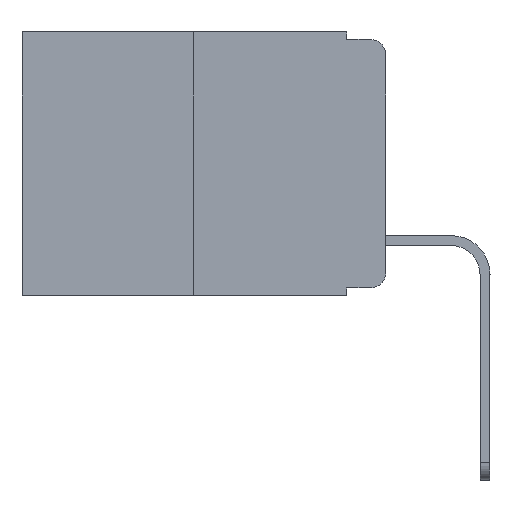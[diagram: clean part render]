
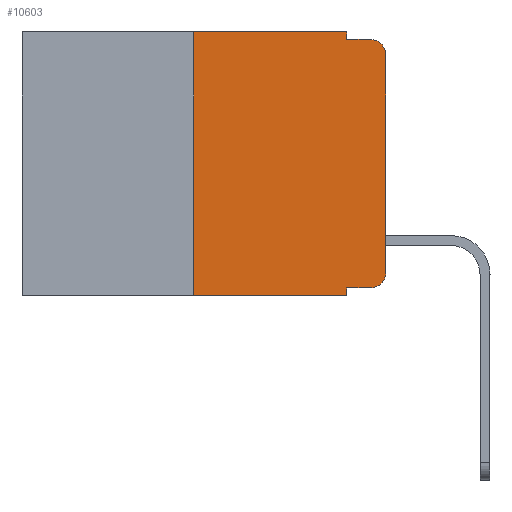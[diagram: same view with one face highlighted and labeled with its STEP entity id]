
A CAD part, left-side view. The second image highlights one B-rep face of the part: STEP entity #10603.
In plain terms, the highlighted planar face has unit normal (-1, 0, 0).
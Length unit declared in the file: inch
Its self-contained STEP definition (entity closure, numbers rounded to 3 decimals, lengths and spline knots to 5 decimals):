
#45 = DIRECTION ( 'NONE',  ( 1., 0., 0. ) ) ;
#70 = CARTESIAN_POINT ( 'NONE',  ( 0., 0.051, -0.343 ) ) ;
#143 = DIRECTION ( 'NONE',  ( 0., 0., -1. ) ) ;
#211 = VECTOR ( 'NONE', #8618, 39.37008 ) ;
#401 = EDGE_CURVE ( 'NONE', #9025, #5847, #8003, .T. ) ;
#471 = CARTESIAN_POINT ( 'NONE',  ( 0., 0.25, 0. ) ) ;
#482 = LINE ( 'NONE', #4358, #211 ) ;
#632 = ORIENTED_EDGE ( 'NONE', *, *, #1402, .T. ) ;
#635 = VERTEX_POINT ( 'NONE', #2144 ) ;
#661 = VECTOR ( 'NONE', #1377, 39.37008 ) ;
#1080 = EDGE_CURVE ( 'NONE', #9693, #635, #1495, .T. ) ;
#1377 = DIRECTION ( 'NONE',  ( 0., 0., 1. ) ) ;
#1402 = EDGE_CURVE ( 'NONE', #5847, #8115, #1760, .T. ) ;
#1495 = LINE ( 'NONE', #10605, #9600 ) ;
#1736 = ORIENTED_EDGE ( 'NONE', *, *, #7422, .F. ) ;
#1760 = LINE ( 'NONE', #5033, #10663 ) ;
#1771 = CARTESIAN_POINT ( 'NONE',  ( 0., 0.473, 0. ) ) ;
#1972 = DIRECTION ( 'NONE',  ( -1., 0., 0. ) ) ;
#2054 = LINE ( 'NONE', #2616, #4363 ) ;
#2144 = CARTESIAN_POINT ( 'NONE',  ( 0., 0.02, -0.01 ) ) ;
#2616 = CARTESIAN_POINT ( 'NONE',  ( 0., 0.051, -0.333 ) ) ;
#2675 = EDGE_LOOP ( 'NONE', ( #632, #10513, #5081, #4228, #2771, #8760, #10245, #1736, #8537, #11148 ) ) ;
#2734 = EDGE_CURVE ( 'NONE', #5361, #9025, #2054, .T. ) ;
#2771 = ORIENTED_EDGE ( 'NONE', *, *, #8094, .F. ) ;
#2781 = EDGE_CURVE ( 'NONE', #10192, #9693, #7338, .T. ) ;
#2884 = AXIS2_PLACEMENT_3D ( 'NONE', #5532, #1972, #4721 ) ;
#2901 = LINE ( 'NONE', #6798, #3985 ) ;
#3283 = FACE_OUTER_BOUND ( 'NONE', #2675, .T. ) ;
#3798 = CARTESIAN_POINT ( 'NONE',  ( 0., 0.02, -0.333 ) ) ;
#3841 = CARTESIAN_POINT ( 'NONE',  ( 0., 0.051, 0. ) ) ;
#3880 = VERTEX_POINT ( 'NONE', #7489 ) ;
#3985 = VECTOR ( 'NONE', #10196, 39.37008 ) ;
#4228 = ORIENTED_EDGE ( 'NONE', *, *, #2781, .F. ) ;
#4239 = CIRCLE ( 'NONE', #2884, 0.02 ) ;
#4358 = CARTESIAN_POINT ( 'NONE',  ( 0., 0.051, 0. ) ) ;
#4363 = VECTOR ( 'NONE', #6846, 39.37008 ) ;
#4426 = DIRECTION ( 'NONE',  ( 0., -1., 0. ) ) ;
#4572 = DIRECTION ( 'NONE',  ( -1., 0., 0. ) ) ;
#4721 = DIRECTION ( 'NONE',  ( 0., 0., -1. ) ) ;
#5033 = CARTESIAN_POINT ( 'NONE',  ( 0., 0., 0. ) ) ;
#5081 = ORIENTED_EDGE ( 'NONE', *, *, #1080, .F. ) ;
#5195 = CARTESIAN_POINT ( 'NONE',  ( 0., 0.051, -0.333 ) ) ;
#5239 = AXIS2_PLACEMENT_3D ( 'NONE', #10438, #4572, #143 ) ;
#5260 = VERTEX_POINT ( 'NONE', #70 ) ;
#5361 = VERTEX_POINT ( 'NONE', #5195 ) ;
#5532 = CARTESIAN_POINT ( 'NONE',  ( 0., 0.02, -0.03 ) ) ;
#5631 = EDGE_CURVE ( 'NONE', #9500, #3880, #8090, .T. ) ;
#5632 = VECTOR ( 'NONE', #4426, 39.37008 ) ;
#5847 = VERTEX_POINT ( 'NONE', #8410 ) ;
#6134 = CARTESIAN_POINT ( 'NONE',  ( 0., 0.473, 0. ) ) ;
#6629 = CARTESIAN_POINT ( 'NONE',  ( 0., 0.051, -0.01 ) ) ;
#6798 = CARTESIAN_POINT ( 'NONE',  ( 0., 0.473, -0.343 ) ) ;
#6846 = DIRECTION ( 'NONE',  ( 0., -1., 0. ) ) ;
#6994 = CARTESIAN_POINT ( 'NONE',  ( 0., 0.051, 0. ) ) ;
#7025 = DIRECTION ( 'NONE',  ( 0., 0., -1. ) ) ;
#7338 = LINE ( 'NONE', #6994, #9633 ) ;
#7422 = EDGE_CURVE ( 'NONE', #5361, #5260, #482, .T. ) ;
#7489 = CARTESIAN_POINT ( 'NONE',  ( 0., 0.25, 0. ) ) ;
#8003 = CIRCLE ( 'NONE', #5239, 0.02 ) ;
#8090 = LINE ( 'NONE', #471, #661 ) ;
#8094 = EDGE_CURVE ( 'NONE', #3880, #10192, #9415, .T. ) ;
#8115 = VERTEX_POINT ( 'NONE', #8641 ) ;
#8198 = AXIS2_PLACEMENT_3D ( 'NONE', #1771, #45, #8721 ) ;
#8410 = CARTESIAN_POINT ( 'NONE',  ( 0., 0., -0.313 ) ) ;
#8537 = ORIENTED_EDGE ( 'NONE', *, *, #2734, .T. ) ;
#8578 = EDGE_CURVE ( 'NONE', #9500, #5260, #2901, .T. ) ;
#8618 = DIRECTION ( 'NONE',  ( 0., 0., -1. ) ) ;
#8641 = CARTESIAN_POINT ( 'NONE',  ( 0., 0., -0.03 ) ) ;
#8721 = DIRECTION ( 'NONE',  ( 0., 0., -1. ) ) ;
#8760 = ORIENTED_EDGE ( 'NONE', *, *, #5631, .F. ) ;
#9025 = VERTEX_POINT ( 'NONE', #3798 ) ;
#9415 = LINE ( 'NONE', #6134, #5632 ) ;
#9500 = VERTEX_POINT ( 'NONE', #10623 ) ;
#9525 = EDGE_CURVE ( 'NONE', #8115, #635, #4239, .T. ) ;
#9600 = VECTOR ( 'NONE', #10647, 39.37008 ) ;
#9633 = VECTOR ( 'NONE', #7025, 39.37008 ) ;
#9693 = VERTEX_POINT ( 'NONE', #6629 ) ;
#10192 = VERTEX_POINT ( 'NONE', #3841 ) ;
#10196 = DIRECTION ( 'NONE',  ( 0., -1., 0. ) ) ;
#10213 = DIRECTION ( 'NONE',  ( 0., 0., 1. ) ) ;
#10245 = ORIENTED_EDGE ( 'NONE', *, *, #8578, .T. ) ;
#10416 = PLANE ( 'NONE',  #8198 ) ;
#10438 = CARTESIAN_POINT ( 'NONE',  ( 0., 0.02, -0.313 ) ) ;
#10513 = ORIENTED_EDGE ( 'NONE', *, *, #9525, .T. ) ;
#10603 = ADVANCED_FACE ( 'NONE', ( #3283 ), #10416, .F. ) ;
#10605 = CARTESIAN_POINT ( 'NONE',  ( 0., 0.051, -0.01 ) ) ;
#10623 = CARTESIAN_POINT ( 'NONE',  ( 0., 0.25, -0.343 ) ) ;
#10647 = DIRECTION ( 'NONE',  ( 0., -1., 0. ) ) ;
#10663 = VECTOR ( 'NONE', #10213, 39.37008 ) ;
#11148 = ORIENTED_EDGE ( 'NONE', *, *, #401, .T. ) ;
